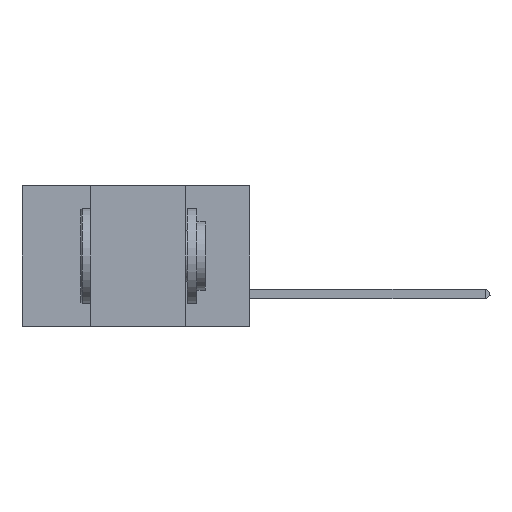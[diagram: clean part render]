
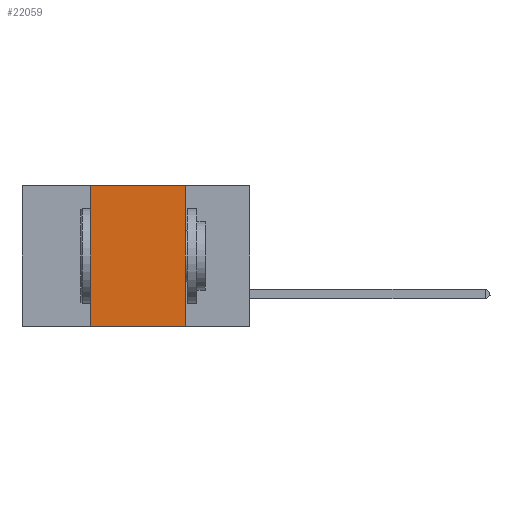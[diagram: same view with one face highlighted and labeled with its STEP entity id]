
A CAD part, left-side view. The second image highlights one B-rep face of the part: STEP entity #22059.
In plain terms, the highlighted planar face has unit normal (-1, 0, 0).
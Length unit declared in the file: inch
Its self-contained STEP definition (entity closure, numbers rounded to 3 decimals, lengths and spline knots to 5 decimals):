
#22 = VERTEX_POINT ( 'NONE', #10667 ) ;
#708 = ORIENTED_EDGE ( 'NONE', *, *, #17489, .F. ) ;
#1198 = LINE ( 'NONE', #18620, #29899 ) ;
#9464 = CARTESIAN_POINT ( 'NONE',  ( 0., 0.6, 0. ) ) ;
#9680 = DIRECTION ( 'NONE',  ( 0., 0., -1. ) ) ;
#9875 = LINE ( 'NONE', #16303, #33283 ) ;
#10667 = CARTESIAN_POINT ( 'NONE',  ( 0., 0.17, 0. ) ) ;
#10963 = CARTESIAN_POINT ( 'NONE',  ( 0., 0.42, 0. ) ) ;
#12076 = LINE ( 'NONE', #47059, #26158 ) ;
#12702 = CARTESIAN_POINT ( 'NONE',  ( 0., 0.17, -0.37 ) ) ;
#14164 = CARTESIAN_POINT ( 'NONE',  ( 0., 0.42, -0.37 ) ) ;
#14862 = DIRECTION ( 'NONE',  ( 0., 0., 1. ) ) ;
#16303 = CARTESIAN_POINT ( 'NONE',  ( 0., 0.6, 0. ) ) ;
#17489 = EDGE_CURVE ( 'NONE', #36450, #35309, #1198, .T. ) ;
#18620 = CARTESIAN_POINT ( 'NONE',  ( 0., 0.42, 0. ) ) ;
#22059 = ADVANCED_FACE ( 'NONE', ( #28537 ), #28159, .F. ) ;
#26158 = VECTOR ( 'NONE', #9680, 39.37008 ) ;
#28101 = DIRECTION ( 'NONE',  ( 0., -1., 0. ) ) ;
#28159 = PLANE ( 'NONE',  #29153 ) ;
#28537 = FACE_OUTER_BOUND ( 'NONE', #47590, .T. ) ;
#29044 = LINE ( 'NONE', #39099, #40757 ) ;
#29153 = AXIS2_PLACEMENT_3D ( 'NONE', #9464, #47174, #46843 ) ;
#29346 = EDGE_CURVE ( 'NONE', #22, #38088, #12076, .T. ) ;
#29899 = VECTOR ( 'NONE', #14862, 39.37008 ) ;
#33283 = VECTOR ( 'NONE', #42715, 39.37008 ) ;
#35309 = VERTEX_POINT ( 'NONE', #10963 ) ;
#36450 = VERTEX_POINT ( 'NONE', #14164 ) ;
#36837 = ORIENTED_EDGE ( 'NONE', *, *, #36878, .T. ) ;
#36878 = EDGE_CURVE ( 'NONE', #36450, #38088, #29044, .T. ) ;
#37707 = ORIENTED_EDGE ( 'NONE', *, *, #47361, .F. ) ;
#38088 = VERTEX_POINT ( 'NONE', #12702 ) ;
#38124 = ORIENTED_EDGE ( 'NONE', *, *, #29346, .F. ) ;
#39099 = CARTESIAN_POINT ( 'NONE',  ( 0., 0.6, -0.37 ) ) ;
#40757 = VECTOR ( 'NONE', #28101, 39.37008 ) ;
#42715 = DIRECTION ( 'NONE',  ( 0., -1., 0. ) ) ;
#46843 = DIRECTION ( 'NONE',  ( 0., 0., -1. ) ) ;
#47059 = CARTESIAN_POINT ( 'NONE',  ( 0., 0.17, 0. ) ) ;
#47174 = DIRECTION ( 'NONE',  ( 1., 0., 0. ) ) ;
#47361 = EDGE_CURVE ( 'NONE', #35309, #22, #9875, .T. ) ;
#47590 = EDGE_LOOP ( 'NONE', ( #38124, #37707, #708, #36837 ) ) ;
